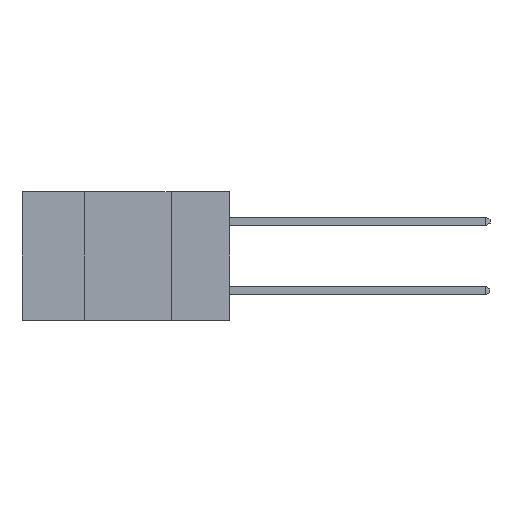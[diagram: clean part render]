
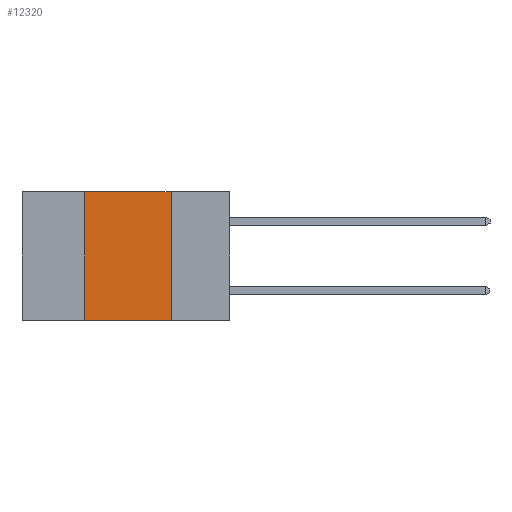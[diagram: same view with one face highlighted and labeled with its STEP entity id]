
A CAD part, left-side view. The second image highlights one B-rep face of the part: STEP entity #12320.
In plain terms, the highlighted planar face has unit normal (-1, 0, 0).
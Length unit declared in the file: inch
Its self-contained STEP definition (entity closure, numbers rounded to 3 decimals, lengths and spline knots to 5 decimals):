
#702 = VERTEX_POINT ( 'NONE', #3040 ) ;
#994 = EDGE_CURVE ( 'NONE', #702, #6805, #5547, .T. ) ;
#1172 = VECTOR ( 'NONE', #12493, 39.37008 ) ;
#1272 = VERTEX_POINT ( 'NONE', #11445 ) ;
#1471 = DIRECTION ( 'NONE',  ( 0., 0., -1. ) ) ;
#1567 = EDGE_LOOP ( 'NONE', ( #4916, #7827, #5256, #8154 ) ) ;
#1816 = LINE ( 'NONE', #3545, #12927 ) ;
#2889 = FACE_OUTER_BOUND ( 'NONE', #1567, .T. ) ;
#3040 = CARTESIAN_POINT ( 'NONE',  ( 0., 0.42, -0.37 ) ) ;
#3471 = DIRECTION ( 'NONE',  ( 0., 0., -1. ) ) ;
#3545 = CARTESIAN_POINT ( 'NONE',  ( 0., 0.17, 0. ) ) ;
#3561 = EDGE_CURVE ( 'NONE', #1272, #6805, #1816, .T. ) ;
#4916 = ORIENTED_EDGE ( 'NONE', *, *, #3561, .F. ) ;
#5202 = DIRECTION ( 'NONE',  ( 0., -1., 0. ) ) ;
#5256 = ORIENTED_EDGE ( 'NONE', *, *, #7893, .F. ) ;
#5547 = LINE ( 'NONE', #6558, #13745 ) ;
#6521 = CARTESIAN_POINT ( 'NONE',  ( 0., 0.42, 0. ) ) ;
#6558 = CARTESIAN_POINT ( 'NONE',  ( 0., 0.6, -0.37 ) ) ;
#6805 = VERTEX_POINT ( 'NONE', #7675 ) ;
#6930 = CARTESIAN_POINT ( 'NONE',  ( 0., 0.6, 0. ) ) ;
#6982 = LINE ( 'NONE', #11440, #1172 ) ;
#7675 = CARTESIAN_POINT ( 'NONE',  ( 0., 0.17, -0.37 ) ) ;
#7827 = ORIENTED_EDGE ( 'NONE', *, *, #8965, .F. ) ;
#7893 = EDGE_CURVE ( 'NONE', #702, #10909, #9316, .T. ) ;
#7984 = DIRECTION ( 'NONE',  ( 1., 0., 0. ) ) ;
#8154 = ORIENTED_EDGE ( 'NONE', *, *, #994, .T. ) ;
#8965 = EDGE_CURVE ( 'NONE', #10909, #1272, #6982, .T. ) ;
#9316 = LINE ( 'NONE', #12903, #12151 ) ;
#9705 = DIRECTION ( 'NONE',  ( 0., 0., 1. ) ) ;
#10909 = VERTEX_POINT ( 'NONE', #6521 ) ;
#11092 = AXIS2_PLACEMENT_3D ( 'NONE', #6930, #7984, #1471 ) ;
#11440 = CARTESIAN_POINT ( 'NONE',  ( 0., 0.6, 0. ) ) ;
#11445 = CARTESIAN_POINT ( 'NONE',  ( 0., 0.17, 0. ) ) ;
#12151 = VECTOR ( 'NONE', #9705, 39.37008 ) ;
#12320 = ADVANCED_FACE ( 'NONE', ( #2889 ), #13280, .F. ) ;
#12493 = DIRECTION ( 'NONE',  ( 0., -1., 0. ) ) ;
#12903 = CARTESIAN_POINT ( 'NONE',  ( 0., 0.42, 0. ) ) ;
#12927 = VECTOR ( 'NONE', #3471, 39.37008 ) ;
#13280 = PLANE ( 'NONE',  #11092 ) ;
#13745 = VECTOR ( 'NONE', #5202, 39.37008 ) ;
